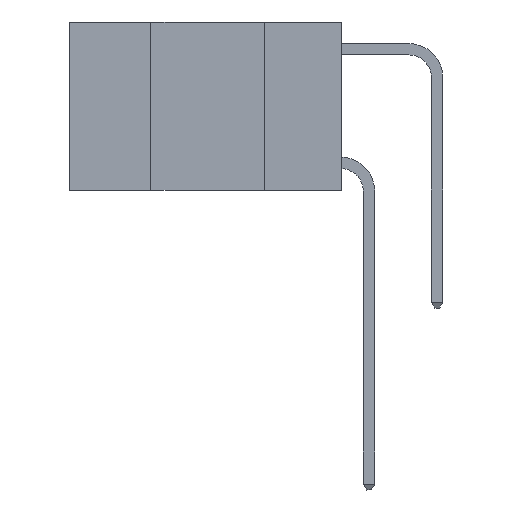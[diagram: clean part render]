
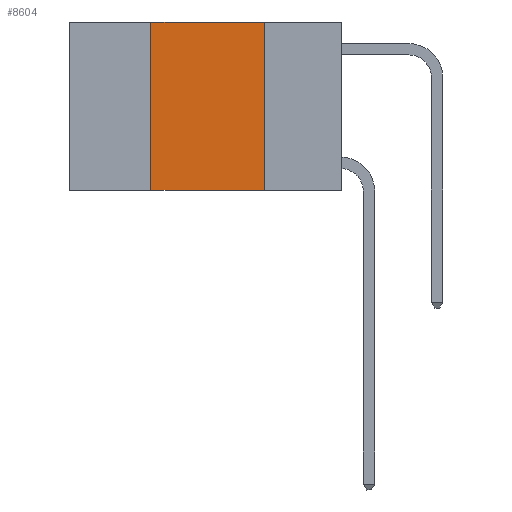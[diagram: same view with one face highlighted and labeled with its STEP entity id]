
A CAD part, left-side view. The second image highlights one B-rep face of the part: STEP entity #8604.
In plain terms, the highlighted planar face has unit normal (-1, 0, 0).
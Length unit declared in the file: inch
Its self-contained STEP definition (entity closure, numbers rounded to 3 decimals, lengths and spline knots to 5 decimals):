
#575 = VECTOR ( 'NONE', #1489, 39.37008 ) ;
#709 = DIRECTION ( 'NONE',  ( 1., 0., 0. ) ) ;
#721 = VERTEX_POINT ( 'NONE', #3767 ) ;
#931 = ORIENTED_EDGE ( 'NONE', *, *, #8304, .F. ) ;
#1258 = CARTESIAN_POINT ( 'NONE',  ( 0., 0.42, -0.37 ) ) ;
#1286 = CARTESIAN_POINT ( 'NONE',  ( 0., 0.6, 0. ) ) ;
#1489 = DIRECTION ( 'NONE',  ( 0., -1., 0. ) ) ;
#1625 = LINE ( 'NONE', #7257, #575 ) ;
#2303 = VECTOR ( 'NONE', #12757, 39.37008 ) ;
#2647 = VERTEX_POINT ( 'NONE', #3164 ) ;
#2654 = LINE ( 'NONE', #7079, #2303 ) ;
#2850 = CARTESIAN_POINT ( 'NONE',  ( 0., 0.42, 0. ) ) ;
#2933 = VERTEX_POINT ( 'NONE', #3972 ) ;
#3164 = CARTESIAN_POINT ( 'NONE',  ( 0., 0.17, 0. ) ) ;
#3767 = CARTESIAN_POINT ( 'NONE',  ( 0., 0.42, 0. ) ) ;
#3956 = FACE_OUTER_BOUND ( 'NONE', #4597, .T. ) ;
#3972 = CARTESIAN_POINT ( 'NONE',  ( 0., 0.17, -0.37 ) ) ;
#4210 = EDGE_CURVE ( 'NONE', #2647, #2933, #2654, .T. ) ;
#4411 = ORIENTED_EDGE ( 'NONE', *, *, #5647, .F. ) ;
#4597 = EDGE_LOOP ( 'NONE', ( #7736, #931, #4411, #13428 ) ) ;
#5078 = DIRECTION ( 'NONE',  ( 0., 0., -1. ) ) ;
#5109 = VERTEX_POINT ( 'NONE', #1258 ) ;
#5379 = VECTOR ( 'NONE', #8580, 39.37008 ) ;
#5647 = EDGE_CURVE ( 'NONE', #5109, #721, #6206, .T. ) ;
#6206 = LINE ( 'NONE', #2850, #8015 ) ;
#7079 = CARTESIAN_POINT ( 'NONE',  ( 0., 0.17, 0. ) ) ;
#7257 = CARTESIAN_POINT ( 'NONE',  ( 0., 0.6, -0.37 ) ) ;
#7286 = EDGE_CURVE ( 'NONE', #5109, #2933, #1625, .T. ) ;
#7736 = ORIENTED_EDGE ( 'NONE', *, *, #4210, .F. ) ;
#8015 = VECTOR ( 'NONE', #8505, 39.37008 ) ;
#8304 = EDGE_CURVE ( 'NONE', #721, #2647, #11715, .T. ) ;
#8503 = CARTESIAN_POINT ( 'NONE',  ( 0., 0.6, 0. ) ) ;
#8505 = DIRECTION ( 'NONE',  ( 0., 0., 1. ) ) ;
#8580 = DIRECTION ( 'NONE',  ( 0., -1., 0. ) ) ;
#8604 = ADVANCED_FACE ( 'NONE', ( #3956 ), #10539, .F. ) ;
#10539 = PLANE ( 'NONE',  #11812 ) ;
#11715 = LINE ( 'NONE', #8503, #5379 ) ;
#11812 = AXIS2_PLACEMENT_3D ( 'NONE', #1286, #709, #5078 ) ;
#12757 = DIRECTION ( 'NONE',  ( 0., 0., -1. ) ) ;
#13428 = ORIENTED_EDGE ( 'NONE', *, *, #7286, .T. ) ;
